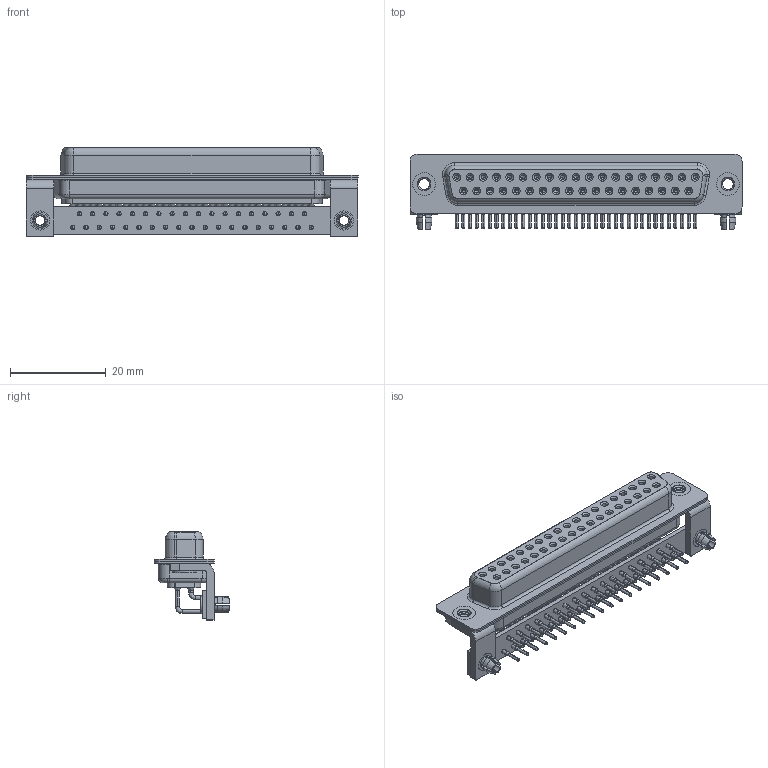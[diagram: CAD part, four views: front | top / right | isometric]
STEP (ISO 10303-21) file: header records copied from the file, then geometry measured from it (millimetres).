
FILE_DESCRIPTION (( 'STEP AP203' ), '1' );
FILE_NAME ('622-M37-660-BN3.STEP', '2018-09-24T22:56:02', ( '' ), ( '' ), 'SwSTEP 2.0', 'SolidWorks 2016', '' );
FILE_SCHEMA (( 'CONFIG_CONTROL_DESIGN' ));
Length unit declared in the file: millimetre
Products named in the file (10): 622M Contact Row 2; 622M 4-40 Threaded Rivet_Stabilizer; 622M Stabilizer Bracket; 622M Stabilizer Board_37 Contacts; 622M Board Lock; 622M Housing_37 Contacts; 622-M37-660-BN3; 622M Shell Front_37 Contacts; 622M Shell Rear_37 Contacts; 622M Contact Row 1
Assembly tree (47 placements, depth 2):
  622-M37-660-BN3
    622M Housing_37 Contacts
    622M Shell Front_37 Contacts
    622M Shell Rear_37 Contacts
    622M Contact Row 1  x19
    622M Contact Row 2  x18
    622M 4-40 Threaded Rivet_Stabilizer  x2
    622M Stabilizer Bracket  x2
    622M Stabilizer Board_37 Contacts
    622M Board Lock  x2
Bounding box: 69.4 x 15.8 x 18.5 mm (x, y, z)
Volume: 6064.5 mm3; surface area: 14973.6 mm2
Topology: 47 solids, 47 shells, 2456 faces, 6278 edges, 3968 vertices
Faces by surface type: cylinder 1116, plane 696, cone 427, bspline 154, torus 63
Entity records: 32237 total; most frequent: CARTESIAN_POINT 6573, DIRECTION 5449, ORIENTED_EDGE 4536, AXIS2_PLACEMENT_3D 2282, EDGE_CURVE 2268, VERTEX_POINT 1455, CIRCLE 1286, EDGE_LOOP 1255
